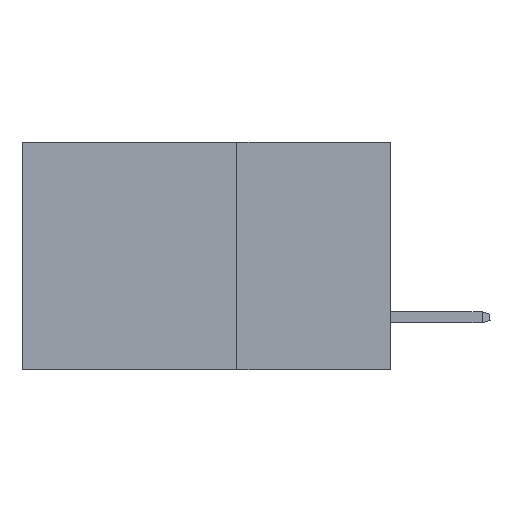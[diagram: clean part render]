
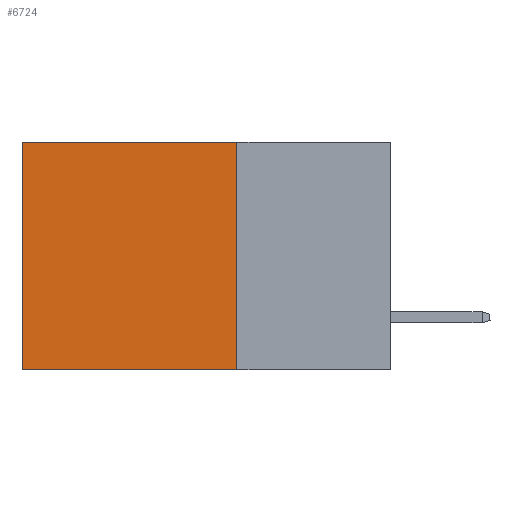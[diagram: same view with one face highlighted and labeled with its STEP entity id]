
A CAD part, left-side view. The second image highlights one B-rep face of the part: STEP entity #6724.
In plain terms, the highlighted planar face has unit normal (-1, 0, 0).
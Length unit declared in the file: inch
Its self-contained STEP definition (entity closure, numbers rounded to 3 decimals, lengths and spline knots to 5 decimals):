
#700 = VERTEX_POINT ( 'NONE', #2306 ) ;
#832 = ORIENTED_EDGE ( 'NONE', *, *, #11973, .T. ) ;
#2306 = CARTESIAN_POINT ( 'NONE',  ( 0.2875, 0.25, -0.37 ) ) ;
#2458 = CARTESIAN_POINT ( 'NONE',  ( 0.2875, 0.25, 0. ) ) ;
#2915 = VERTEX_POINT ( 'NONE', #13778 ) ;
#3207 = DIRECTION ( 'NONE',  ( 0., 1., 0. ) ) ;
#3496 = PLANE ( 'NONE',  #16238 ) ;
#4084 = LINE ( 'NONE', #4868, #9787 ) ;
#4363 = EDGE_LOOP ( 'NONE', ( #4403, #13175, #11091, #832 ) ) ;
#4403 = ORIENTED_EDGE ( 'NONE', *, *, #15809, .T. ) ;
#4612 = VERTEX_POINT ( 'NONE', #12013 ) ;
#4644 = FACE_OUTER_BOUND ( 'NONE', #4363, .T. ) ;
#4839 = DIRECTION ( 'NONE',  ( 0., 0., -1. ) ) ;
#4868 = CARTESIAN_POINT ( 'NONE',  ( 0.2875, 0.25, -0.37 ) ) ;
#5837 = EDGE_CURVE ( 'NONE', #700, #6470, #4084, .T. ) ;
#6106 = DIRECTION ( 'NONE',  ( 0., 0., -1. ) ) ;
#6470 = VERTEX_POINT ( 'NONE', #11712 ) ;
#6724 = ADVANCED_FACE ( 'NONE', ( #4644 ), #3496, .F. ) ;
#7634 = LINE ( 'NONE', #8148, #9792 ) ;
#8148 = CARTESIAN_POINT ( 'NONE',  ( 0.2875, 0.25, 0. ) ) ;
#8601 = CARTESIAN_POINT ( 'NONE',  ( 0.2875, 0.25, 0. ) ) ;
#9166 = LINE ( 'NONE', #2458, #14254 ) ;
#9787 = VECTOR ( 'NONE', #9892, 39.37008 ) ;
#9792 = VECTOR ( 'NONE', #3207, 39.37008 ) ;
#9892 = DIRECTION ( 'NONE',  ( 0., 1., 0. ) ) ;
#10427 = VECTOR ( 'NONE', #4839, 39.37008 ) ;
#11075 = CARTESIAN_POINT ( 'NONE',  ( 0.2875, 0.6, 0. ) ) ;
#11091 = ORIENTED_EDGE ( 'NONE', *, *, #12978, .F. ) ;
#11712 = CARTESIAN_POINT ( 'NONE',  ( 0.2875, 0.6, -0.37 ) ) ;
#11973 = EDGE_CURVE ( 'NONE', #2915, #4612, #7634, .T. ) ;
#12013 = CARTESIAN_POINT ( 'NONE',  ( 0.2875, 0.6, 0. ) ) ;
#12294 = DIRECTION ( 'NONE',  ( 0., 0., -1. ) ) ;
#12978 = EDGE_CURVE ( 'NONE', #2915, #700, #9166, .T. ) ;
#13175 = ORIENTED_EDGE ( 'NONE', *, *, #5837, .F. ) ;
#13778 = CARTESIAN_POINT ( 'NONE',  ( 0.2875, 0.25, 0. ) ) ;
#14254 = VECTOR ( 'NONE', #12294, 39.37008 ) ;
#14528 = LINE ( 'NONE', #11075, #10427 ) ;
#15809 = EDGE_CURVE ( 'NONE', #4612, #6470, #14528, .T. ) ;
#15969 = DIRECTION ( 'NONE',  ( 1., 0., 0. ) ) ;
#16238 = AXIS2_PLACEMENT_3D ( 'NONE', #8601, #15969, #6106 ) ;
